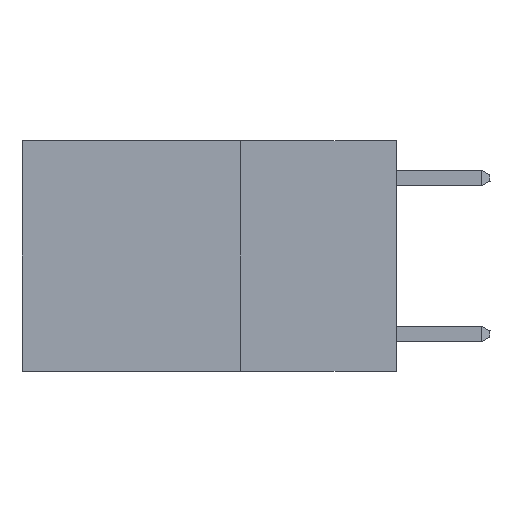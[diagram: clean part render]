
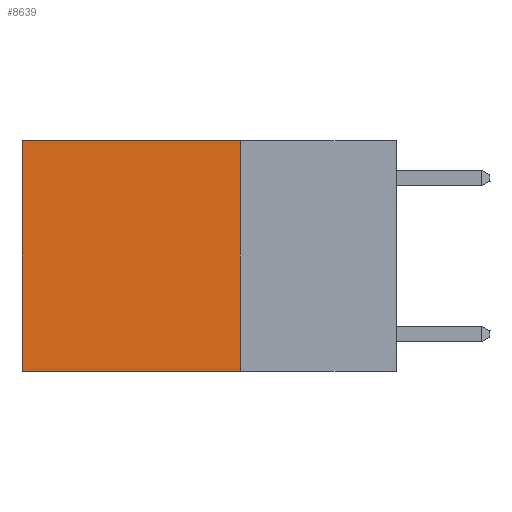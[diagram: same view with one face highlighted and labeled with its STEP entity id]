
A CAD part, left-side view. The second image highlights one B-rep face of the part: STEP entity #8639.
In plain terms, the highlighted planar face has unit normal (-1, 0, 0).
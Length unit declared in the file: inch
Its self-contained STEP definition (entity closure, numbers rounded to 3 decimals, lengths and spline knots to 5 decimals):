
#141 = VECTOR ( 'NONE', #10789, 39.37008 ) ;
#979 = EDGE_CURVE ( 'NONE', #3182, #10731, #18617, .T. ) ;
#2001 = CARTESIAN_POINT ( 'NONE',  ( 0.2625, 0.25, 0. ) ) ;
#2455 = PLANE ( 'NONE',  #7091 ) ;
#3182 = VERTEX_POINT ( 'NONE', #20581 ) ;
#3325 = ORIENTED_EDGE ( 'NONE', *, *, #16007, .F. ) ;
#3937 = ORIENTED_EDGE ( 'NONE', *, *, #18209, .F. ) ;
#4473 = CARTESIAN_POINT ( 'NONE',  ( 0.2625, 0.25, 0. ) ) ;
#4586 = VERTEX_POINT ( 'NONE', #17596 ) ;
#4895 = DIRECTION ( 'NONE',  ( 0., 1., 0. ) ) ;
#6519 = CARTESIAN_POINT ( 'NONE',  ( 0.2625, 0.25, -0.37 ) ) ;
#6714 = VECTOR ( 'NONE', #4895, 39.37008 ) ;
#7091 = AXIS2_PLACEMENT_3D ( 'NONE', #4473, #8935, #24427 ) ;
#8107 = VERTEX_POINT ( 'NONE', #6519 ) ;
#8639 = ADVANCED_FACE ( 'NONE', ( #13816 ), #2455, .F. ) ;
#8935 = DIRECTION ( 'NONE',  ( 1., 0., 0. ) ) ;
#9487 = CARTESIAN_POINT ( 'NONE',  ( 0.2625, 0.25, 0. ) ) ;
#9734 = LINE ( 'NONE', #12198, #16884 ) ;
#10033 = DIRECTION ( 'NONE',  ( 0., 0., -1. ) ) ;
#10731 = VERTEX_POINT ( 'NONE', #18583 ) ;
#10789 = DIRECTION ( 'NONE',  ( 0., 0., -1. ) ) ;
#11712 = EDGE_CURVE ( 'NONE', #10731, #4586, #9734, .T. ) ;
#12198 = CARTESIAN_POINT ( 'NONE',  ( 0.2625, 0.6, 0. ) ) ;
#13482 = ORIENTED_EDGE ( 'NONE', *, *, #11712, .T. ) ;
#13816 = FACE_OUTER_BOUND ( 'NONE', #17483, .T. ) ;
#14617 = CARTESIAN_POINT ( 'NONE',  ( 0.2625, 0.25, -0.37 ) ) ;
#16007 = EDGE_CURVE ( 'NONE', #3182, #8107, #19107, .T. ) ;
#16884 = VECTOR ( 'NONE', #10033, 39.37008 ) ;
#17041 = LINE ( 'NONE', #14617, #24683 ) ;
#17483 = EDGE_LOOP ( 'NONE', ( #13482, #3937, #3325, #20860 ) ) ;
#17596 = CARTESIAN_POINT ( 'NONE',  ( 0.2625, 0.6, -0.37 ) ) ;
#18209 = EDGE_CURVE ( 'NONE', #8107, #4586, #17041, .T. ) ;
#18583 = CARTESIAN_POINT ( 'NONE',  ( 0.2625, 0.6, 0. ) ) ;
#18617 = LINE ( 'NONE', #9487, #6714 ) ;
#19107 = LINE ( 'NONE', #2001, #141 ) ;
#20581 = CARTESIAN_POINT ( 'NONE',  ( 0.2625, 0.25, 0. ) ) ;
#20860 = ORIENTED_EDGE ( 'NONE', *, *, #979, .T. ) ;
#24427 = DIRECTION ( 'NONE',  ( 0., 0., -1. ) ) ;
#24683 = VECTOR ( 'NONE', #25953, 39.37008 ) ;
#25953 = DIRECTION ( 'NONE',  ( 0., 1., 0. ) ) ;
